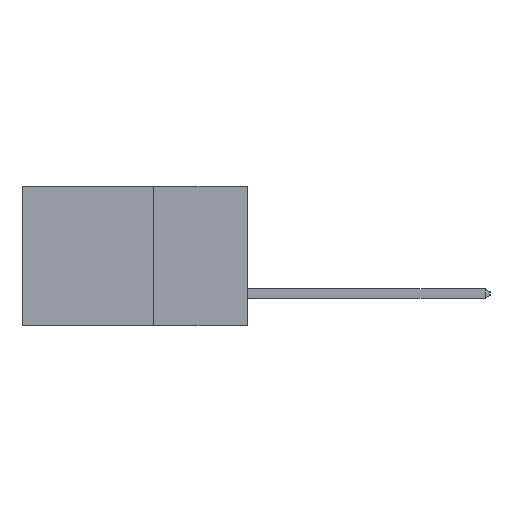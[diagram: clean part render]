
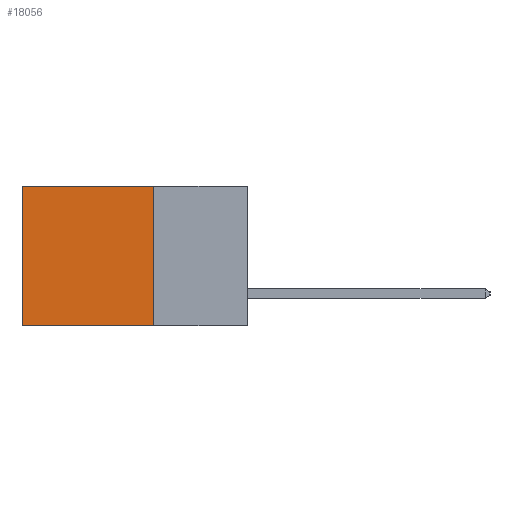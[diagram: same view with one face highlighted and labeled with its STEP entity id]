
A CAD part, left-side view. The second image highlights one B-rep face of the part: STEP entity #18056.
In plain terms, the highlighted planar face has unit normal (-1, 0, 0).
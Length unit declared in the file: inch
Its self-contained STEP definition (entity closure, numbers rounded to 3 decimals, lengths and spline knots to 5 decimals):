
#4418 = ORIENTED_EDGE ( 'NONE', *, *, #16796, .F. ) ;
#4640 = EDGE_CURVE ( 'NONE', #11698, #20610, #6642, .T. ) ;
#5881 = VECTOR ( 'NONE', #19170, 39.37008 ) ;
#6642 = LINE ( 'NONE', #12762, #20154 ) ;
#6759 = LINE ( 'NONE', #16993, #25096 ) ;
#7049 = DIRECTION ( 'NONE',  ( 0., 0., -1. ) ) ;
#8464 = ORIENTED_EDGE ( 'NONE', *, *, #23998, .F. ) ;
#8664 = FACE_OUTER_BOUND ( 'NONE', #20979, .T. ) ;
#11698 = VERTEX_POINT ( 'NONE', #22198 ) ;
#12762 = CARTESIAN_POINT ( 'NONE',  ( 0.298, 0.6, 0. ) ) ;
#12961 = LINE ( 'NONE', #28973, #25019 ) ;
#16517 = CARTESIAN_POINT ( 'NONE',  ( 0.298, 0.25, 0. ) ) ;
#16690 = CARTESIAN_POINT ( 'NONE',  ( 0.298, 0.25, 0. ) ) ;
#16796 = EDGE_CURVE ( 'NONE', #29969, #20954, #24935, .T. ) ;
#16993 = CARTESIAN_POINT ( 'NONE',  ( 0.298, 0.25, 0. ) ) ;
#17408 = DIRECTION ( 'NONE',  ( 0., 0., -1. ) ) ;
#18056 = ADVANCED_FACE ( 'NONE', ( #8664 ), #19003, .F. ) ;
#18794 = CARTESIAN_POINT ( 'NONE',  ( 0.298, 0.25, 0. ) ) ;
#19003 = PLANE ( 'NONE',  #25774 ) ;
#19170 = DIRECTION ( 'NONE',  ( 0., 0., -1. ) ) ;
#19497 = DIRECTION ( 'NONE',  ( 0., 1., 0. ) ) ;
#20154 = VECTOR ( 'NONE', #17408, 39.37008 ) ;
#20565 = ORIENTED_EDGE ( 'NONE', *, *, #28907, .T. ) ;
#20610 = VERTEX_POINT ( 'NONE', #21930 ) ;
#20954 = VERTEX_POINT ( 'NONE', #25482 ) ;
#20979 = EDGE_LOOP ( 'NONE', ( #24655, #8464, #4418, #20565 ) ) ;
#21448 = DIRECTION ( 'NONE',  ( 1., 0., 0. ) ) ;
#21930 = CARTESIAN_POINT ( 'NONE',  ( 0.298, 0.6, -0.37 ) ) ;
#22198 = CARTESIAN_POINT ( 'NONE',  ( 0.298, 0.6, 0. ) ) ;
#23998 = EDGE_CURVE ( 'NONE', #20954, #20610, #12961, .T. ) ;
#24468 = DIRECTION ( 'NONE',  ( 0., 1., 0. ) ) ;
#24655 = ORIENTED_EDGE ( 'NONE', *, *, #4640, .T. ) ;
#24935 = LINE ( 'NONE', #16690, #5881 ) ;
#25019 = VECTOR ( 'NONE', #24468, 39.37008 ) ;
#25096 = VECTOR ( 'NONE', #19497, 39.37008 ) ;
#25482 = CARTESIAN_POINT ( 'NONE',  ( 0.298, 0.25, -0.37 ) ) ;
#25774 = AXIS2_PLACEMENT_3D ( 'NONE', #18794, #21448, #7049 ) ;
#28907 = EDGE_CURVE ( 'NONE', #29969, #11698, #6759, .T. ) ;
#28973 = CARTESIAN_POINT ( 'NONE',  ( 0.298, 0.25, -0.37 ) ) ;
#29969 = VERTEX_POINT ( 'NONE', #16517 ) ;
